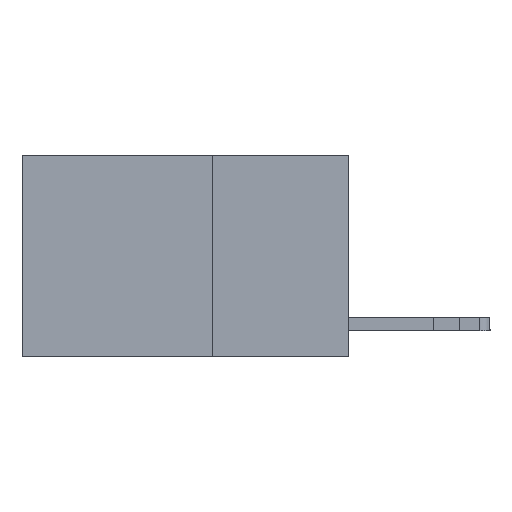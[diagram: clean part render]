
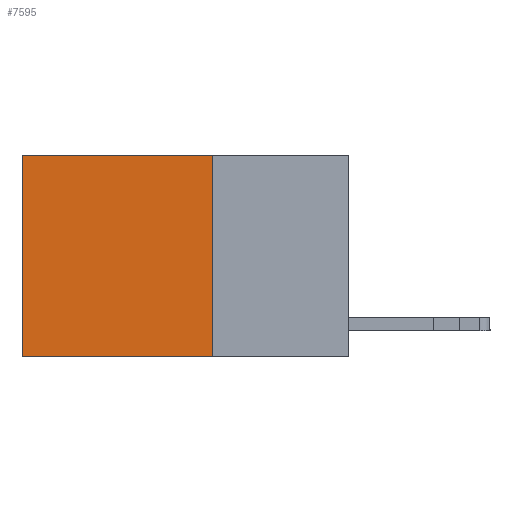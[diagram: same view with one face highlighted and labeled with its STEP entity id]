
A CAD part, left-side view. The second image highlights one B-rep face of the part: STEP entity #7595.
In plain terms, the highlighted planar face has unit normal (-1, 0, 0).
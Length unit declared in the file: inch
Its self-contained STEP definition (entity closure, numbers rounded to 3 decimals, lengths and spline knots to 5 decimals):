
#1117 = CARTESIAN_POINT ( 'NONE',  ( 0.2625, 0.25, 0. ) ) ;
#2905 = CARTESIAN_POINT ( 'NONE',  ( 0.2625, 0.25, -0.37 ) ) ;
#4015 = EDGE_LOOP ( 'NONE', ( #11353, #14677, #7629, #11183 ) ) ;
#4048 = EDGE_CURVE ( 'NONE', #12316, #11902, #14141, .T. ) ;
#4847 = VECTOR ( 'NONE', #5238, 39.37008 ) ;
#5238 = DIRECTION ( 'NONE',  ( 0., 1., 0. ) ) ;
#6205 = VECTOR ( 'NONE', #9067, 39.37008 ) ;
#6237 = CARTESIAN_POINT ( 'NONE',  ( 0.2625, 0.6, 0. ) ) ;
#6498 = EDGE_CURVE ( 'NONE', #8528, #11902, #9720, .T. ) ;
#6697 = FACE_OUTER_BOUND ( 'NONE', #4015, .T. ) ;
#7258 = VECTOR ( 'NONE', #14292, 39.37008 ) ;
#7595 = ADVANCED_FACE ( 'NONE', ( #6697 ), #9082, .F. ) ;
#7629 = ORIENTED_EDGE ( 'NONE', *, *, #11291, .F. ) ;
#7779 = LINE ( 'NONE', #7930, #9543 ) ;
#7930 = CARTESIAN_POINT ( 'NONE',  ( 0.2625, 0.25, 0. ) ) ;
#8528 = VERTEX_POINT ( 'NONE', #14626 ) ;
#8604 = CARTESIAN_POINT ( 'NONE',  ( 0.2625, 0.6, 0. ) ) ;
#9067 = DIRECTION ( 'NONE',  ( 0., 1., 0. ) ) ;
#9082 = PLANE ( 'NONE',  #11122 ) ;
#9543 = VECTOR ( 'NONE', #12324, 39.37008 ) ;
#9720 = LINE ( 'NONE', #2905, #4847 ) ;
#10209 = CARTESIAN_POINT ( 'NONE',  ( 0.2625, 0.25, 0. ) ) ;
#10929 = VERTEX_POINT ( 'NONE', #1117 ) ;
#11122 = AXIS2_PLACEMENT_3D ( 'NONE', #10209, #11243, #12508 ) ;
#11183 = ORIENTED_EDGE ( 'NONE', *, *, #12092, .T. ) ;
#11243 = DIRECTION ( 'NONE',  ( 1., 0., 0. ) ) ;
#11291 = EDGE_CURVE ( 'NONE', #10929, #8528, #7779, .T. ) ;
#11353 = ORIENTED_EDGE ( 'NONE', *, *, #4048, .T. ) ;
#11902 = VERTEX_POINT ( 'NONE', #12072 ) ;
#12072 = CARTESIAN_POINT ( 'NONE',  ( 0.2625, 0.6, -0.37 ) ) ;
#12092 = EDGE_CURVE ( 'NONE', #10929, #12316, #12637, .T. ) ;
#12316 = VERTEX_POINT ( 'NONE', #8604 ) ;
#12324 = DIRECTION ( 'NONE',  ( 0., 0., -1. ) ) ;
#12508 = DIRECTION ( 'NONE',  ( 0., 0., -1. ) ) ;
#12637 = LINE ( 'NONE', #13684, #6205 ) ;
#13684 = CARTESIAN_POINT ( 'NONE',  ( 0.2625, 0.25, 0. ) ) ;
#14141 = LINE ( 'NONE', #6237, #7258 ) ;
#14292 = DIRECTION ( 'NONE',  ( 0., 0., -1. ) ) ;
#14626 = CARTESIAN_POINT ( 'NONE',  ( 0.2625, 0.25, -0.37 ) ) ;
#14677 = ORIENTED_EDGE ( 'NONE', *, *, #6498, .F. ) ;
